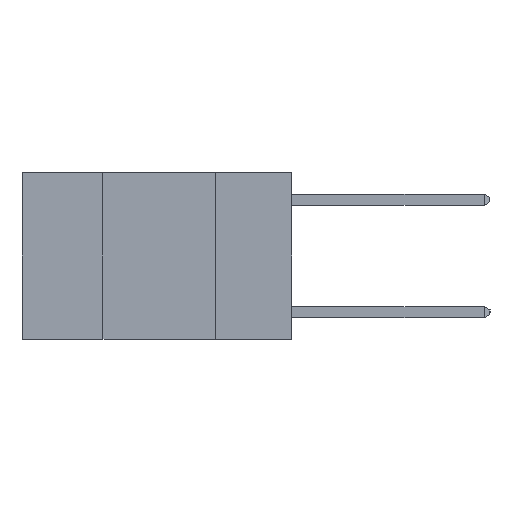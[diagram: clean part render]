
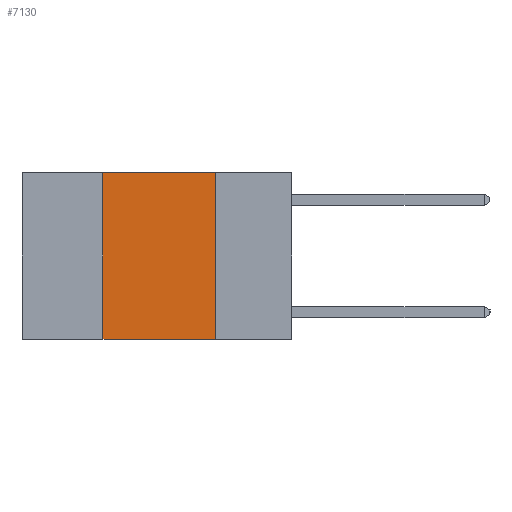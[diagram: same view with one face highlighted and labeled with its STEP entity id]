
A CAD part, left-side view. The second image highlights one B-rep face of the part: STEP entity #7130.
In plain terms, the highlighted planar face has unit normal (-1, 0, 0).
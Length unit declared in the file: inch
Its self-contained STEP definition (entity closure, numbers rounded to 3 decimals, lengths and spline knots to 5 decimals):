
#93 = DIRECTION ( 'NONE',  ( 0., 0., 1. ) ) ;
#1779 = VERTEX_POINT ( 'NONE', #6746 ) ;
#1925 = CARTESIAN_POINT ( 'NONE',  ( 0., 0.6, 0. ) ) ;
#2367 = VECTOR ( 'NONE', #2989, 39.37008 ) ;
#2602 = LINE ( 'NONE', #5988, #9550 ) ;
#2652 = CARTESIAN_POINT ( 'NONE',  ( 0., 0.42, -0.37 ) ) ;
#2658 = LINE ( 'NONE', #3951, #2367 ) ;
#2875 = VERTEX_POINT ( 'NONE', #5683 ) ;
#2884 = DIRECTION ( 'NONE',  ( 0., -1., 0. ) ) ;
#2979 = EDGE_CURVE ( 'NONE', #9978, #1779, #2658, .T. ) ;
#2989 = DIRECTION ( 'NONE',  ( 0., -1., 0. ) ) ;
#3065 = FACE_OUTER_BOUND ( 'NONE', #5911, .T. ) ;
#3402 = CARTESIAN_POINT ( 'NONE',  ( 0., 0.42, 0. ) ) ;
#3715 = ORIENTED_EDGE ( 'NONE', *, *, #2979, .T. ) ;
#3951 = CARTESIAN_POINT ( 'NONE',  ( 0., 0.6, -0.37 ) ) ;
#3956 = CARTESIAN_POINT ( 'NONE',  ( 0., 0.6, 0. ) ) ;
#4689 = EDGE_CURVE ( 'NONE', #2875, #1779, #10216, .T. ) ;
#4916 = DIRECTION ( 'NONE',  ( 1., 0., 0. ) ) ;
#5209 = VECTOR ( 'NONE', #12274, 39.37008 ) ;
#5683 = CARTESIAN_POINT ( 'NONE',  ( 0., 0.17, 0. ) ) ;
#5911 = EDGE_LOOP ( 'NONE', ( #6072, #7023, #10034, #3715 ) ) ;
#5988 = CARTESIAN_POINT ( 'NONE',  ( 0., 0.42, 0. ) ) ;
#6072 = ORIENTED_EDGE ( 'NONE', *, *, #4689, .F. ) ;
#6746 = CARTESIAN_POINT ( 'NONE',  ( 0., 0.17, -0.37 ) ) ;
#7023 = ORIENTED_EDGE ( 'NONE', *, *, #8846, .F. ) ;
#7031 = AXIS2_PLACEMENT_3D ( 'NONE', #3956, #4916, #11485 ) ;
#7130 = ADVANCED_FACE ( 'NONE', ( #3065 ), #9612, .F. ) ;
#7854 = EDGE_CURVE ( 'NONE', #9978, #11142, #2602, .T. ) ;
#8084 = LINE ( 'NONE', #1925, #10541 ) ;
#8846 = EDGE_CURVE ( 'NONE', #11142, #2875, #8084, .T. ) ;
#9550 = VECTOR ( 'NONE', #93, 39.37008 ) ;
#9612 = PLANE ( 'NONE',  #7031 ) ;
#9636 = CARTESIAN_POINT ( 'NONE',  ( 0., 0.17, 0. ) ) ;
#9978 = VERTEX_POINT ( 'NONE', #2652 ) ;
#10034 = ORIENTED_EDGE ( 'NONE', *, *, #7854, .F. ) ;
#10216 = LINE ( 'NONE', #9636, #5209 ) ;
#10541 = VECTOR ( 'NONE', #2884, 39.37008 ) ;
#11142 = VERTEX_POINT ( 'NONE', #3402 ) ;
#11485 = DIRECTION ( 'NONE',  ( 0., 0., -1. ) ) ;
#12274 = DIRECTION ( 'NONE',  ( 0., 0., -1. ) ) ;
